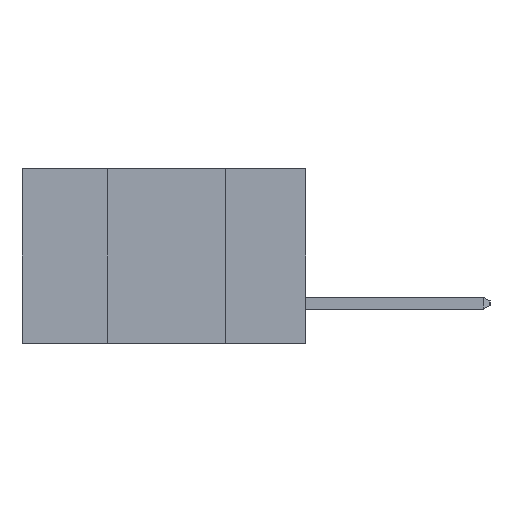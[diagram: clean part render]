
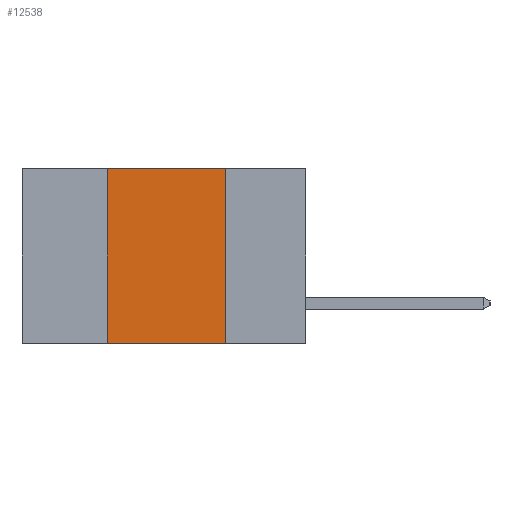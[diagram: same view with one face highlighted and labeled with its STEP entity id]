
A CAD part, left-side view. The second image highlights one B-rep face of the part: STEP entity #12538.
In plain terms, the highlighted planar face has unit normal (-1, 0, 0).
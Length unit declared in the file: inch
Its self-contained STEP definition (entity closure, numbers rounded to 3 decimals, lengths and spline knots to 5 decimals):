
#2249 = CARTESIAN_POINT ( 'NONE',  ( 0., 0.42, -0.37 ) ) ;
#2412 = VECTOR ( 'NONE', #12636, 39.37008 ) ;
#2950 = EDGE_LOOP ( 'NONE', ( #8962, #10034, #12984, #15759 ) ) ;
#3072 = CARTESIAN_POINT ( 'NONE',  ( 0., 0.6, 0. ) ) ;
#3931 = EDGE_CURVE ( 'NONE', #5933, #12700, #14358, .T. ) ;
#3938 = CARTESIAN_POINT ( 'NONE',  ( 0., 0.6, 0. ) ) ;
#3943 = AXIS2_PLACEMENT_3D ( 'NONE', #3938, #12608, #5217 ) ;
#4640 = LINE ( 'NONE', #3072, #14061 ) ;
#4674 = LINE ( 'NONE', #9369, #10511 ) ;
#5217 = DIRECTION ( 'NONE',  ( 0., 0., -1. ) ) ;
#5492 = CARTESIAN_POINT ( 'NONE',  ( 0., 0.17, 0. ) ) ;
#5800 = LINE ( 'NONE', #11444, #2412 ) ;
#5933 = VERTEX_POINT ( 'NONE', #2249 ) ;
#8711 = EDGE_CURVE ( 'NONE', #15117, #15201, #5800, .T. ) ;
#8962 = ORIENTED_EDGE ( 'NONE', *, *, #8711, .F. ) ;
#9307 = DIRECTION ( 'NONE',  ( 0., -1., 0. ) ) ;
#9367 = EDGE_CURVE ( 'NONE', #12700, #15117, #4640, .T. ) ;
#9369 = CARTESIAN_POINT ( 'NONE',  ( 0., 0.6, -0.37 ) ) ;
#9499 = DIRECTION ( 'NONE',  ( 0., 0., 1. ) ) ;
#9623 = CARTESIAN_POINT ( 'NONE',  ( 0., 0.42, -0.37 ) ) ;
#10034 = ORIENTED_EDGE ( 'NONE', *, *, #9367, .F. ) ;
#10511 = VECTOR ( 'NONE', #15359, 39.37008 ) ;
#10604 = CARTESIAN_POINT ( 'NONE',  ( 0., 0.17, -0.37 ) ) ;
#11165 = VECTOR ( 'NONE', #9499, 39.37008 ) ;
#11444 = CARTESIAN_POINT ( 'NONE',  ( 0., 0.17, -0.37 ) ) ;
#12300 = FACE_OUTER_BOUND ( 'NONE', #2950, .T. ) ;
#12503 = PLANE ( 'NONE',  #3943 ) ;
#12538 = ADVANCED_FACE ( 'NONE', ( #12300 ), #12503, .F. ) ;
#12608 = DIRECTION ( 'NONE',  ( 1., 0., 0. ) ) ;
#12636 = DIRECTION ( 'NONE',  ( 0., 0., -1. ) ) ;
#12700 = VERTEX_POINT ( 'NONE', #14122 ) ;
#12984 = ORIENTED_EDGE ( 'NONE', *, *, #3931, .F. ) ;
#14061 = VECTOR ( 'NONE', #9307, 39.37008 ) ;
#14122 = CARTESIAN_POINT ( 'NONE',  ( 0., 0.42, 0. ) ) ;
#14358 = LINE ( 'NONE', #9623, #11165 ) ;
#14563 = EDGE_CURVE ( 'NONE', #5933, #15201, #4674, .T. ) ;
#15117 = VERTEX_POINT ( 'NONE', #5492 ) ;
#15201 = VERTEX_POINT ( 'NONE', #10604 ) ;
#15359 = DIRECTION ( 'NONE',  ( 0., -1., 0. ) ) ;
#15759 = ORIENTED_EDGE ( 'NONE', *, *, #14563, .T. ) ;
